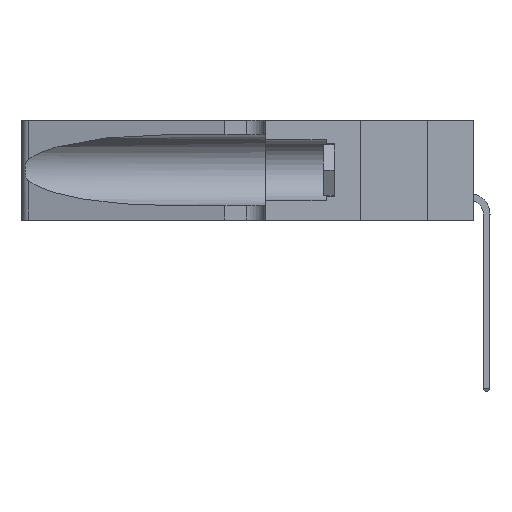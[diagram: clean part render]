
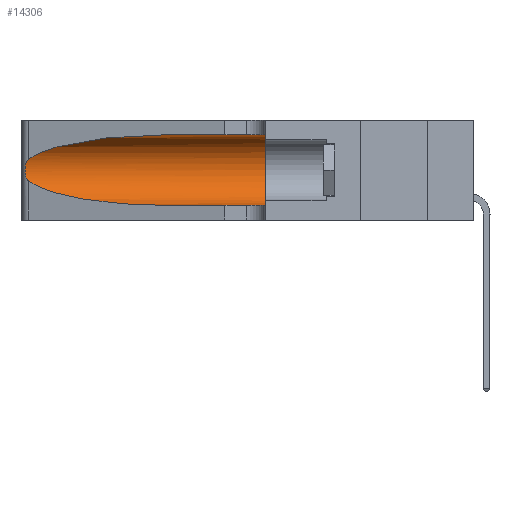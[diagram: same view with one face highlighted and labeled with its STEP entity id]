
A CAD part, left-side view. The second image highlights one B-rep face of the part: STEP entity #14306.
In plain terms, the highlighted cylindrical face has radius 3.308 mm (diameter 6.617 mm), a partial arc.
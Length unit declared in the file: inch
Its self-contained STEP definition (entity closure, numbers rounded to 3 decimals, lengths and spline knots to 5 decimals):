
#170 = CARTESIAN_POINT ( 'NONE',  ( 0.25487, 1.22718, 0.14631 ) ) ;
#382 = CARTESIAN_POINT ( 'NONE',  ( 0.18966, 0.96281, 0.31525 ) ) ;
#434 = CARTESIAN_POINT ( 'NONE',  ( 0.26017, 1.23833, 0.17102 ) ) ;
#476 = DIRECTION ( 'NONE',  ( 0., 0., 1. ) ) ;
#743 = ORIENTED_EDGE ( 'NONE', *, *, #18669, .T. ) ;
#878 = CARTESIAN_POINT ( 'NONE',  ( 0.1305, 0.72297, 0.05475 ) ) ;
#1668 = ORIENTED_EDGE ( 'NONE', *, *, #13324, .T. ) ;
#2456 = EDGE_CURVE ( 'NONE', #13932, #27952, #13443, .T. ) ;
#2687 =( BOUNDED_CURVE ( )  B_SPLINE_CURVE ( 3, ( #10683, #24498, #26694, #28993 ),
 .UNSPECIFIED., .F., .T. ) 
 B_SPLINE_CURVE_WITH_KNOTS ( ( 4, 4 ),
 ( 3.44316, 4.71239 ),
 .UNSPECIFIED. ) 
 CURVE ( )  GEOMETRIC_REPRESENTATION_ITEM ( )  RATIONAL_B_SPLINE_CURVE ( ( 1., 0.87, 0.87, 1. ) ) 
 REPRESENTATION_ITEM ( '' )  );
#4724 = CARTESIAN_POINT ( 'NONE',  ( 0.25856, 1.23593, 0.16098 ) ) ;
#4820 = CARTESIAN_POINT ( 'NONE',  ( 0.25487, 1.22718, 0.22369 ) ) ;
#5033 = CARTESIAN_POINT ( 'NONE',  ( 0.25639, 1.23186, 0.15144 ) ) ;
#5435 = CARTESIAN_POINT ( 'NONE',  ( 0.1305, 0.35, 0.31525 ) ) ;
#7000 = ORIENTED_EDGE ( 'NONE', *, *, #2456, .T. ) ;
#7034 = DIRECTION ( 'NONE',  ( 0., -1., 0. ) ) ;
#7500 =( BOUNDED_CURVE ( )  B_SPLINE_CURVE ( 3, ( #14103, #382, #23847, #10117 ),
 .UNSPECIFIED., .F., .F. ) 
 B_SPLINE_CURVE_WITH_KNOTS ( ( 4, 4 ),
 ( 1.5708, 2.84003 ),
 .UNSPECIFIED. ) 
 CURVE ( )  GEOMETRIC_REPRESENTATION_ITEM ( )  RATIONAL_B_SPLINE_CURVE ( ( 1., 0.87, 0.87, 1. ) ) 
 REPRESENTATION_ITEM ( '' )  );
#9350 = CARTESIAN_POINT ( 'NONE',  ( 0.25639, 1.23184, 0.21858 ) ) ;
#9517 = AXIS2_PLACEMENT_3D ( 'NONE', #18459, #7034, #11572 ) ;
#9589 = DIRECTION ( 'NONE',  ( 0., 1., 0. ) ) ;
#10117 = CARTESIAN_POINT ( 'NONE',  ( 0.25487, 1.22718, 0.22369 ) ) ;
#10683 = CARTESIAN_POINT ( 'NONE',  ( 0.25487, 1.22718, 0.14631 ) ) ;
#10878 = EDGE_CURVE ( 'NONE', #25842, #13932, #2687, .T. ) ;
#11572 = DIRECTION ( 'NONE',  ( 0., 0., -1. ) ) ;
#11875 = CARTESIAN_POINT ( 'NONE',  ( 0.25787, 1.23484, 0.2124 ) ) ;
#12621 = CARTESIAN_POINT ( 'NONE',  ( 0.1305, 0.72297, 0.31525 ) ) ;
#13293 = CARTESIAN_POINT ( 'NONE',  ( 0.1305, 1.61858, 0.05475 ) ) ;
#13324 = EDGE_CURVE ( 'NONE', #22200, #25842, #25677, .T. ) ;
#13443 = LINE ( 'NONE', #13293, #25262 ) ;
#13574 = AXIS2_PLACEMENT_3D ( 'NONE', #27911, #9589, #476 ) ;
#13932 = VERTEX_POINT ( 'NONE', #878 ) ;
#13962 = CARTESIAN_POINT ( 'NONE',  ( 0.25789, 1.23486, 0.15765 ) ) ;
#14103 = CARTESIAN_POINT ( 'NONE',  ( 0.1305, 0.72297, 0.31525 ) ) ;
#14164 = CARTESIAN_POINT ( 'NONE',  ( 0.26018, 1.23835, 0.19895 ) ) ;
#14306 = ADVANCED_FACE ( 'NONE', ( #18224 ), #22193, .F. ) ;
#14359 = CARTESIAN_POINT ( 'NONE',  ( 0.26075, 1.23896, 0.178 ) ) ;
#16353 = CARTESIAN_POINT ( 'NONE',  ( 0.25555, 1.22994, 0.2215 ) ) ;
#17060 = CARTESIAN_POINT ( 'NONE',  ( 0.25487, 1.22718, 0.22369 ) ) ;
#17207 = ORIENTED_EDGE ( 'NONE', *, *, #24199, .F. ) ;
#18224 = FACE_OUTER_BOUND ( 'NONE', #24735, .T. ) ;
#18292 = ORIENTED_EDGE ( 'NONE', *, *, #28354, .F. ) ;
#18459 = CARTESIAN_POINT ( 'NONE',  ( 0.1305, 1.61858, 0.185 ) ) ;
#18651 = CARTESIAN_POINT ( 'NONE',  ( 0.26075, 1.23896, 0.19203 ) ) ;
#18669 = EDGE_CURVE ( 'NONE', #21866, #22200, #7500, .T. ) ;
#19980 = DIRECTION ( 'NONE',  ( 0., -1., 0. ) ) ;
#20029 = CARTESIAN_POINT ( 'NONE',  ( 0.1305, 0.35, 0.05475 ) ) ;
#21068 = CARTESIAN_POINT ( 'NONE',  ( 0.25555, 1.22993, 0.14849 ) ) ;
#21866 = VERTEX_POINT ( 'NONE', #12621 ) ;
#22193 = CYLINDRICAL_SURFACE ( 'NONE', #9517, 0.13025 ) ;
#22200 = VERTEX_POINT ( 'NONE', #17060 ) ;
#23375 = CARTESIAN_POINT ( 'NONE',  ( 0.25487, 1.22718, 0.14631 ) ) ;
#23642 = DIRECTION ( 'NONE',  ( 0., -1., 0. ) ) ;
#23847 = CARTESIAN_POINT ( 'NONE',  ( 0.2373, 1.15595, 0.28018 ) ) ;
#23946 = VERTEX_POINT ( 'NONE', #5435 ) ;
#24199 = EDGE_CURVE ( 'NONE', #21866, #23946, #28166, .T. ) ;
#24252 = VECTOR ( 'NONE', #23642, 39.37008 ) ;
#24344 = CIRCLE ( 'NONE', #13574, 0.13025 ) ;
#24498 = CARTESIAN_POINT ( 'NONE',  ( 0.2373, 1.15595, 0.08982 ) ) ;
#24735 = EDGE_LOOP ( 'NONE', ( #743, #1668, #26291, #7000, #18292, #17207 ) ) ;
#25262 = VECTOR ( 'NONE', #19980, 39.37008 ) ;
#25677 = B_SPLINE_CURVE_WITH_KNOTS ( 'NONE', 3,
 ( #4820, #16353, #9350, #11875, #27679, #14164, #18651, #14359, #434, #4724, #13962, #5033, #21068, #23375 ),
 .UNSPECIFIED., .F., .F.,
 ( 4, 2, 2, 2, 2, 2, 4 ),
 ( 0., 0.00027, 0.00053, 0.00107, 0.0016, 0.00187, 0.00214 ),
 .UNSPECIFIED. ) ;
#25842 = VERTEX_POINT ( 'NONE', #170 ) ;
#26291 = ORIENTED_EDGE ( 'NONE', *, *, #10878, .T. ) ;
#26694 = CARTESIAN_POINT ( 'NONE',  ( 0.18966, 0.96281, 0.05475 ) ) ;
#27679 = CARTESIAN_POINT ( 'NONE',  ( 0.25854, 1.2359, 0.20912 ) ) ;
#27911 = CARTESIAN_POINT ( 'NONE',  ( 0.1305, 0.35, 0.185 ) ) ;
#27952 = VERTEX_POINT ( 'NONE', #20029 ) ;
#28043 = CARTESIAN_POINT ( 'NONE',  ( 0.1305, 1.61858, 0.31525 ) ) ;
#28166 = LINE ( 'NONE', #28043, #24252 ) ;
#28354 = EDGE_CURVE ( 'NONE', #23946, #27952, #24344, .T. ) ;
#28993 = CARTESIAN_POINT ( 'NONE',  ( 0.1305, 0.72297, 0.05475 ) ) ;
